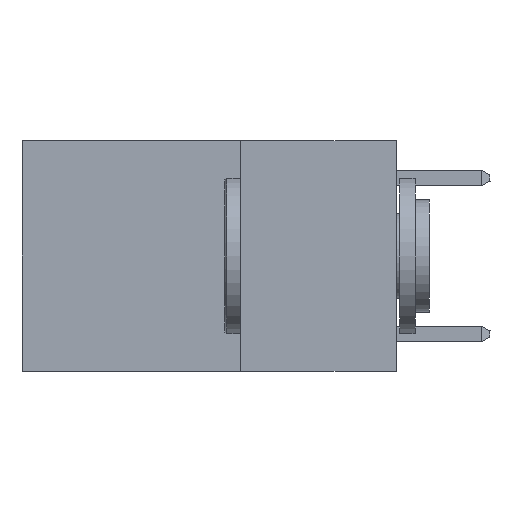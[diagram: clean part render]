
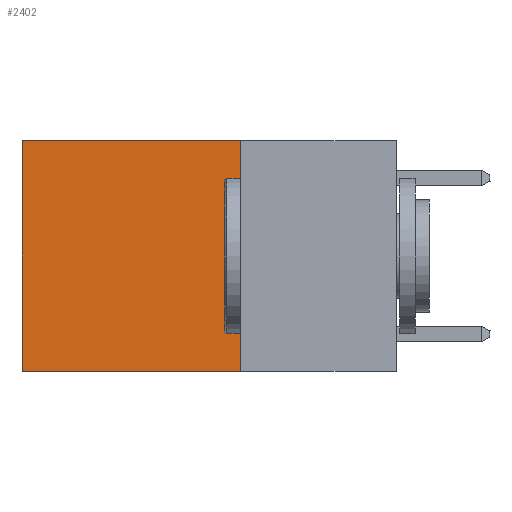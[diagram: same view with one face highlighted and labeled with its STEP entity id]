
A CAD part, left-side view. The second image highlights one B-rep face of the part: STEP entity #2402.
In plain terms, the highlighted planar face has unit normal (-1, 0, 0).
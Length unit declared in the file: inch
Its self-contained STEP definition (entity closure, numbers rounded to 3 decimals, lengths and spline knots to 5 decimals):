
#440 = VERTEX_POINT ( 'NONE', #24488 ) ;
#1828 = CARTESIAN_POINT ( 'NONE',  ( 0.2625, 0.25, -0.37 ) ) ;
#2402 = ADVANCED_FACE ( 'NONE', ( #4187 ), #8100, .F. ) ;
#2769 = VERTEX_POINT ( 'NONE', #11686 ) ;
#4187 = FACE_OUTER_BOUND ( 'NONE', #13814, .T. ) ;
#4475 = ORIENTED_EDGE ( 'NONE', *, *, #14960, .F. ) ;
#4698 = EDGE_CURVE ( 'NONE', #26527, #440, #8181, .T. ) ;
#5030 = VERTEX_POINT ( 'NONE', #12873 ) ;
#6027 = ORIENTED_EDGE ( 'NONE', *, *, #22764, .T. ) ;
#7133 = CARTESIAN_POINT ( 'NONE',  ( 0.2625, 0.25, 0. ) ) ;
#8100 = PLANE ( 'NONE',  #15619 ) ;
#8181 = LINE ( 'NONE', #1828, #18118 ) ;
#8328 = DIRECTION ( 'NONE',  ( 0., 1., 0. ) ) ;
#8802 = LINE ( 'NONE', #25858, #12300 ) ;
#9445 = DIRECTION ( 'NONE',  ( 0., 1., 0. ) ) ;
#9480 = EDGE_CURVE ( 'NONE', #2769, #5030, #17982, .T. ) ;
#11686 = CARTESIAN_POINT ( 'NONE',  ( 0.2625, 0.25, 0. ) ) ;
#11927 = VECTOR ( 'NONE', #9445, 39.37008 ) ;
#12300 = VECTOR ( 'NONE', #17899, 39.37008 ) ;
#12873 = CARTESIAN_POINT ( 'NONE',  ( 0.2625, 0.6, 0. ) ) ;
#13814 = EDGE_LOOP ( 'NONE', ( #6027, #20910, #4475, #21394 ) ) ;
#14960 = EDGE_CURVE ( 'NONE', #2769, #26527, #20781, .T. ) ;
#15564 = CARTESIAN_POINT ( 'NONE',  ( 0.2625, 0.25, -0.37 ) ) ;
#15619 = AXIS2_PLACEMENT_3D ( 'NONE', #23378, #28155, #16915 ) ;
#16751 = DIRECTION ( 'NONE',  ( 0., 0., -1. ) ) ;
#16915 = DIRECTION ( 'NONE',  ( 0., 0., -1. ) ) ;
#17899 = DIRECTION ( 'NONE',  ( 0., 0., -1. ) ) ;
#17982 = LINE ( 'NONE', #7133, #11927 ) ;
#18118 = VECTOR ( 'NONE', #8328, 39.37008 ) ;
#20781 = LINE ( 'NONE', #25127, #26187 ) ;
#20910 = ORIENTED_EDGE ( 'NONE', *, *, #4698, .F. ) ;
#21394 = ORIENTED_EDGE ( 'NONE', *, *, #9480, .T. ) ;
#22764 = EDGE_CURVE ( 'NONE', #5030, #440, #8802, .T. ) ;
#23378 = CARTESIAN_POINT ( 'NONE',  ( 0.2625, 0.25, 0. ) ) ;
#24488 = CARTESIAN_POINT ( 'NONE',  ( 0.2625, 0.6, -0.37 ) ) ;
#25127 = CARTESIAN_POINT ( 'NONE',  ( 0.2625, 0.25, 0. ) ) ;
#25858 = CARTESIAN_POINT ( 'NONE',  ( 0.2625, 0.6, 0. ) ) ;
#26187 = VECTOR ( 'NONE', #16751, 39.37008 ) ;
#26527 = VERTEX_POINT ( 'NONE', #15564 ) ;
#28155 = DIRECTION ( 'NONE',  ( 1., 0., 0. ) ) ;
